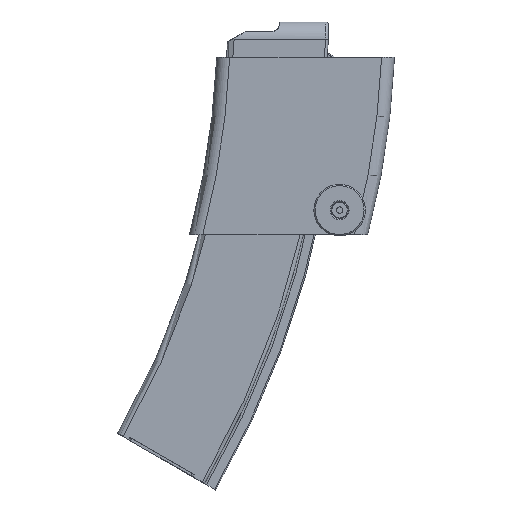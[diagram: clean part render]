
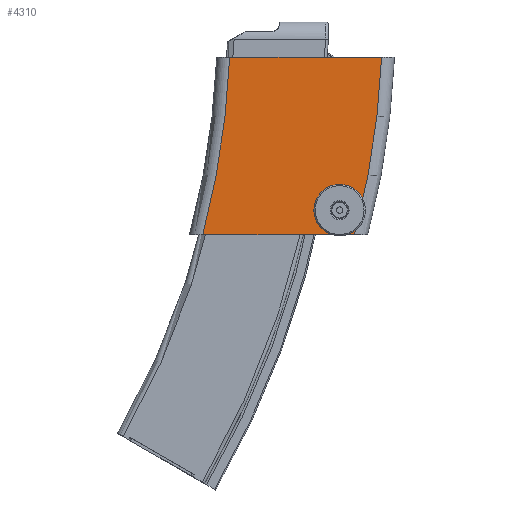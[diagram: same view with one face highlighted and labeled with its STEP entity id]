
A CAD part, front view. The second image highlights one B-rep face of the part: STEP entity #4310.
In plain terms, the highlighted planar face has unit normal (0, -1, 0).
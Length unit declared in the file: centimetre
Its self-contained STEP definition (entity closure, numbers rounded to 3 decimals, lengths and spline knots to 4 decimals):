
#160=LINE($,#7488,#417);
#177=LINE($,#7651,#434);
#186=LINE($,#7674,#443);
#204=LINE($,#8235,#461);
#224=LINE($,#8679,#481);
#226=LINE($,#8732,#483);
#417=VECTOR($,#5288,5.8861);
#434=VECTOR($,#5315,1.29);
#443=VECTOR($,#5336,0.58);
#461=VECTOR($,#5414,1.29);
#481=VECTOR($,#5524,0.68);
#483=VECTOR($,#5546,5.8996);
#835=PLANE($,#4687);
#983=FACE_BOUND($,#1404,.T.);
#1122=FACE_OUTER_BOUND($,#1403,.T.);
#1403=EDGE_LOOP($,(#3458,#3459,#3460,#3461));
#1404=EDGE_LOOP($,(#3462,#3463,#3464,#3465,#3466,#3467));
#1604=CIRCLE($,#4601,0.05);
#1643=CIRCLE($,#4679,0.05);
#1645=CIRCLE($,#4682,32.1);
#1648=CIRCLE($,#4688,32.5);
#1871=VERTEX_POINT($,#7467);
#1873=VERTEX_POINT($,#7487);
#1899=VERTEX_POINT($,#7648);
#1900=VERTEX_POINT($,#7650);
#1906=VERTEX_POINT($,#7666);
#1908=VERTEX_POINT($,#7672);
#1948=VERTEX_POINT($,#8232);
#1949=VERTEX_POINT($,#8234);
#1976=VERTEX_POINT($,#8685);
#1979=VERTEX_POINT($,#8731);
#2352=EDGE_CURVE($,#1873,#1871,#160,.T.);
#2380=EDGE_CURVE($,#1900,#1899,#177,.T.);
#2389=EDGE_CURVE($,#1899,#1906,#1604,.T.);
#2392=EDGE_CURVE($,#1906,#1908,#186,.T.);
#2447=EDGE_CURVE($,#1949,#1948,#204,.T.);
#2504=EDGE_CURVE($,#1948,#1900,#224,.T.);
#2505=EDGE_CURVE($,#1908,#1949,#1643,.T.);
#2508=EDGE_CURVE($,#1976,#1871,#1645,.T.);
#2513=EDGE_CURVE($,#1976,#1979,#226,.F.);
#2514=EDGE_CURVE($,#1873,#1979,#1648,.T.);
#3458=ORIENTED_EDGE($,*,*,#2508,.F.);
#3459=ORIENTED_EDGE($,*,*,#2513,.T.);
#3460=ORIENTED_EDGE($,*,*,#2514,.F.);
#3461=ORIENTED_EDGE($,*,*,#2352,.T.);
#3462=ORIENTED_EDGE($,*,*,#2389,.T.);
#3463=ORIENTED_EDGE($,*,*,#2392,.T.);
#3464=ORIENTED_EDGE($,*,*,#2505,.T.);
#3465=ORIENTED_EDGE($,*,*,#2447,.T.);
#3466=ORIENTED_EDGE($,*,*,#2504,.T.);
#3467=ORIENTED_EDGE($,*,*,#2380,.T.);
#4310=ADVANCED_FACE($,(#1122,#983),#835,.F.);
#4601=AXIS2_PLACEMENT_3D($,#7668,#5330,#5331);
#4679=AXIS2_PLACEMENT_3D($,#8681,#5527,#5528);
#4682=AXIS2_PLACEMENT_3D($,#8704,#5533,#5534);
#4687=AXIS2_PLACEMENT_3D($,#8730,#5544,#5545);
#4688=AXIS2_PLACEMENT_3D($,#8733,#5547,#5548);
#5288=DIRECTION($,(1.,0.,0.));
#5315=DIRECTION($,(1.,0.,0.));
#5330=DIRECTION('center_axis',(0.,1.,0.));
#5331=DIRECTION('ref_axis',(0.707,0.,0.707));
#5336=DIRECTION($,(0.,0.,-1.));
#5414=DIRECTION($,(-1.,0.,0.));
#5524=DIRECTION($,(0.,0.,1.));
#5527=DIRECTION('center_axis',(0.,1.,0.));
#5528=DIRECTION('ref_axis',(0.707,0.,-0.707));
#5533=DIRECTION('center_axis',(0.,1.,0.));
#5534=DIRECTION('ref_axis',(0.989,0.,-0.149));
#5544=DIRECTION('center_axis',(0.,1.,0.));
#5545=DIRECTION('ref_axis',(0.,0.,1.));
#5546=DIRECTION($,(1.,0.,0.));
#5547=DIRECTION('center_axis',(0.,-1.,0.));
#5548=DIRECTION('ref_axis',(0.988,0.,-0.152));
#7467=CARTESIAN_POINT('',(-14.2239,18.2103,9.1));
#7487=CARTESIAN_POINT('',(-20.1101,18.2103,9.1));
#7488=CARTESIAN_POINT($,(-16.5892,18.2103,9.1));
#7648=CARTESIAN_POINT('',(-14.1765,18.2103,10.3933));
#7650=CARTESIAN_POINT('',(-15.4665,18.2103,10.3933));
#7651=CARTESIAN_POINT($,(-15.6531,18.2103,10.3933));
#7666=CARTESIAN_POINT('',(-14.1265,18.2103,10.3433));
#7668=CARTESIAN_POINT('Origin',(-14.1765,18.2103,10.3433));
#7672=CARTESIAN_POINT('',(-14.1265,18.2103,9.7633));
#7674=CARTESIAN_POINT($,(-14.1265,18.2103,10.8766));
#8232=CARTESIAN_POINT('',(-15.4665,18.2103,9.7133));
#8234=CARTESIAN_POINT('',(-14.1765,18.2103,9.7133));
#8235=CARTESIAN_POINT($,(-15.6531,18.2103,9.7133));
#8679=CARTESIAN_POINT($,(-15.4665,18.2103,10.8766));
#8681=CARTESIAN_POINT('Origin',(-14.1765,18.2103,9.7633));
#8685=CARTESIAN_POINT('',(-13.1655,18.2103,16.));
#8704=CARTESIAN_POINT('Origin',(-45.2354,18.2103,17.3884));
#8730=CARTESIAN_POINT('Origin',(-16.2397,18.2103,11.7));
#8731=CARTESIAN_POINT('',(-19.0651,18.2103,16.));
#8732=CARTESIAN_POINT($,(-15.943,18.2103,16.));
#8733=CARTESIAN_POINT('Origin',(-51.5354,18.2103,17.3884));
